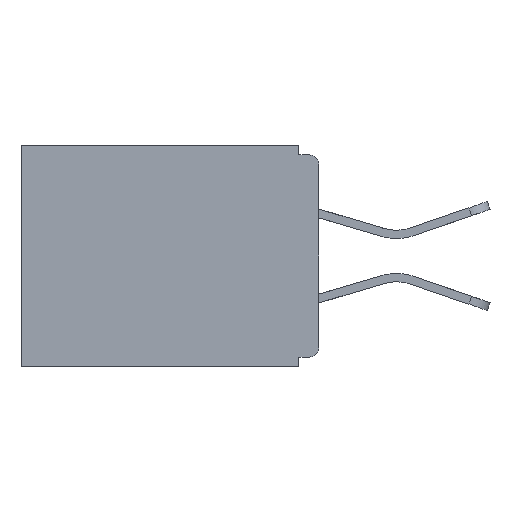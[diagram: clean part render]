
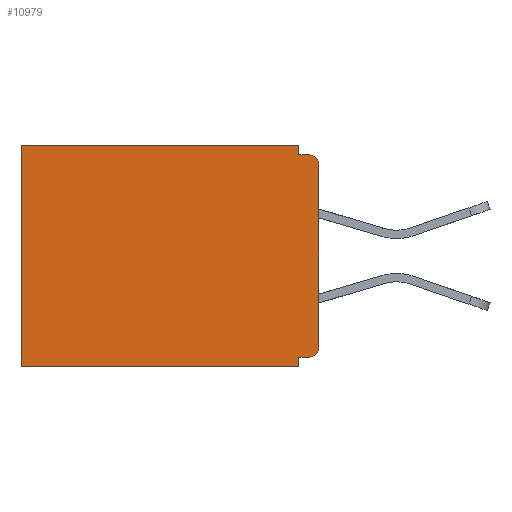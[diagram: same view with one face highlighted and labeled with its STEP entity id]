
A CAD part, left-side view. The second image highlights one B-rep face of the part: STEP entity #10979.
In plain terms, the highlighted planar face has unit normal (-1, 0, 0).
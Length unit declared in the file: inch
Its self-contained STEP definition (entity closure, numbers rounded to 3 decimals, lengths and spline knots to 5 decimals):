
#209 = CARTESIAN_POINT ( 'NONE',  ( 0.298, 0., 0. ) ) ;
#227 = ORIENTED_EDGE ( 'NONE', *, *, #17039, .T. ) ;
#592 = LINE ( 'NONE', #7194, #16999 ) ;
#690 = EDGE_CURVE ( 'NONE', #20075, #6422, #6167, .T. ) ;
#1209 = CARTESIAN_POINT ( 'NONE',  ( 0.298, 0.46, -0.343 ) ) ;
#1606 = EDGE_CURVE ( 'NONE', #6919, #14593, #592, .T. ) ;
#1772 = ORIENTED_EDGE ( 'NONE', *, *, #690, .T. ) ;
#1932 = DIRECTION ( 'NONE',  ( 0., 0., -1. ) ) ;
#1971 = CARTESIAN_POINT ( 'NONE',  ( 0.298, 0., -0.328 ) ) ;
#2287 = DIRECTION ( 'NONE',  ( 0., 0., -1. ) ) ;
#2556 = LINE ( 'NONE', #24312, #23766 ) ;
#2982 = CARTESIAN_POINT ( 'NONE',  ( 0.298, 0., 0. ) ) ;
#3265 = ORIENTED_EDGE ( 'NONE', *, *, #5584, .F. ) ;
#4301 = CARTESIAN_POINT ( 'NONE',  ( 0.298, 0.015, -0.03 ) ) ;
#4576 = VECTOR ( 'NONE', #20540, 39.37008 ) ;
#4629 = DIRECTION ( 'NONE',  ( 0., 0., -1. ) ) ;
#4659 = EDGE_CURVE ( 'NONE', #20075, #15726, #24919, .T. ) ;
#4704 = CARTESIAN_POINT ( 'NONE',  ( 0.298, 0.031, 0. ) ) ;
#5392 = FACE_OUTER_BOUND ( 'NONE', #14101, .T. ) ;
#5584 = EDGE_CURVE ( 'NONE', #16088, #6422, #20590, .T. ) ;
#5958 = ORIENTED_EDGE ( 'NONE', *, *, #4659, .F. ) ;
#6167 = CIRCLE ( 'NONE', #26015, 0.015 ) ;
#6249 = CARTESIAN_POINT ( 'NONE',  ( 0.298, 0.46, 0. ) ) ;
#6354 = VECTOR ( 'NONE', #13911, 39.37008 ) ;
#6369 = ORIENTED_EDGE ( 'NONE', *, *, #21008, .T. ) ;
#6422 = VERTEX_POINT ( 'NONE', #22270 ) ;
#6476 = CARTESIAN_POINT ( 'NONE',  ( 0.298, 0., -0.015 ) ) ;
#6669 = CARTESIAN_POINT ( 'NONE',  ( 0.298, 0.015, -0.328 ) ) ;
#6919 = VERTEX_POINT ( 'NONE', #22104 ) ;
#7194 = CARTESIAN_POINT ( 'NONE',  ( 0.298, 0., -0.343 ) ) ;
#7736 = VERTEX_POINT ( 'NONE', #6249 ) ;
#7957 = LINE ( 'NONE', #23876, #6354 ) ;
#8005 = LINE ( 'NONE', #2982, #18879 ) ;
#9027 = VERTEX_POINT ( 'NONE', #17617 ) ;
#10189 = DIRECTION ( 'NONE',  ( 0., 0., -1. ) ) ;
#10411 = DIRECTION ( 'NONE',  ( 0., 1., 0. ) ) ;
#10531 = PLANE ( 'NONE',  #12973 ) ;
#10979 = ADVANCED_FACE ( 'NONE', ( #5392 ), #10531, .F. ) ;
#11213 = LINE ( 'NONE', #6476, #12820 ) ;
#11377 = VECTOR ( 'NONE', #10411, 39.37008 ) ;
#11609 = CARTESIAN_POINT ( 'NONE',  ( 0.298, 0.031, -0.015 ) ) ;
#12205 = ORIENTED_EDGE ( 'NONE', *, *, #13034, .T. ) ;
#12239 = CARTESIAN_POINT ( 'NONE',  ( 0.298, 0.015, -0.313 ) ) ;
#12820 = VECTOR ( 'NONE', #18508, 39.37008 ) ;
#12973 = AXIS2_PLACEMENT_3D ( 'NONE', #209, #14638, #16970 ) ;
#13034 = EDGE_CURVE ( 'NONE', #16088, #9027, #21733, .T. ) ;
#13911 = DIRECTION ( 'NONE',  ( 0., 0., -1. ) ) ;
#14101 = EDGE_LOOP ( 'NONE', ( #12205, #18159, #20805, #227, #6369, #18441, #16629, #5958, #1772, #3265 ) ) ;
#14593 = VERTEX_POINT ( 'NONE', #1209 ) ;
#14638 = DIRECTION ( 'NONE',  ( 1., 0., 0. ) ) ;
#14910 = EDGE_CURVE ( 'NONE', #15726, #6919, #21263, .T. ) ;
#15726 = VERTEX_POINT ( 'NONE', #17563 ) ;
#16088 = VERTEX_POINT ( 'NONE', #19944 ) ;
#16100 = EDGE_CURVE ( 'NONE', #24744, #9027, #11213, .T. ) ;
#16577 = CARTESIAN_POINT ( 'NONE',  ( 0.298, 0.031, -0.343 ) ) ;
#16629 = ORIENTED_EDGE ( 'NONE', *, *, #14910, .F. ) ;
#16892 = VERTEX_POINT ( 'NONE', #4704 ) ;
#16970 = DIRECTION ( 'NONE',  ( 0., 0., -1. ) ) ;
#16999 = VECTOR ( 'NONE', #25496, 39.37008 ) ;
#17039 = EDGE_CURVE ( 'NONE', #16892, #7736, #8005, .T. ) ;
#17346 = DIRECTION ( 'NONE',  ( 0., 1., 0. ) ) ;
#17563 = CARTESIAN_POINT ( 'NONE',  ( 0.298, 0.031, -0.328 ) ) ;
#17617 = CARTESIAN_POINT ( 'NONE',  ( 0.298, 0.015, -0.015 ) ) ;
#18159 = ORIENTED_EDGE ( 'NONE', *, *, #16100, .F. ) ;
#18441 = ORIENTED_EDGE ( 'NONE', *, *, #1606, .F. ) ;
#18508 = DIRECTION ( 'NONE',  ( 0., -1., 0. ) ) ;
#18729 = CARTESIAN_POINT ( 'NONE',  ( 0.298, 0., 0. ) ) ;
#18879 = VECTOR ( 'NONE', #17346, 39.37008 ) ;
#19264 = VECTOR ( 'NONE', #2287, 39.37008 ) ;
#19934 = AXIS2_PLACEMENT_3D ( 'NONE', #4301, #24936, #4629 ) ;
#19944 = CARTESIAN_POINT ( 'NONE',  ( 0.298, 0., -0.03 ) ) ;
#20075 = VERTEX_POINT ( 'NONE', #6669 ) ;
#20540 = DIRECTION ( 'NONE',  ( 0., 0., -1. ) ) ;
#20590 = LINE ( 'NONE', #18729, #19264 ) ;
#20805 = ORIENTED_EDGE ( 'NONE', *, *, #22495, .F. ) ;
#21008 = EDGE_CURVE ( 'NONE', #7736, #14593, #2556, .T. ) ;
#21263 = LINE ( 'NONE', #16577, #4576 ) ;
#21733 = CIRCLE ( 'NONE', #19934, 0.015 ) ;
#22104 = CARTESIAN_POINT ( 'NONE',  ( 0.298, 0.031, -0.343 ) ) ;
#22270 = CARTESIAN_POINT ( 'NONE',  ( 0.298, 0., -0.313 ) ) ;
#22495 = EDGE_CURVE ( 'NONE', #16892, #24744, #7957, .T. ) ;
#23766 = VECTOR ( 'NONE', #1932, 39.37008 ) ;
#23876 = CARTESIAN_POINT ( 'NONE',  ( 0.298, 0.031, -0.343 ) ) ;
#24312 = CARTESIAN_POINT ( 'NONE',  ( 0.298, 0.46, 0. ) ) ;
#24744 = VERTEX_POINT ( 'NONE', #11609 ) ;
#24919 = LINE ( 'NONE', #1971, #11377 ) ;
#24936 = DIRECTION ( 'NONE',  ( -1., 0., 0. ) ) ;
#25496 = DIRECTION ( 'NONE',  ( 0., 1., 0. ) ) ;
#26015 = AXIS2_PLACEMENT_3D ( 'NONE', #12239, #26518, #10189 ) ;
#26518 = DIRECTION ( 'NONE',  ( -1., 0., 0. ) ) ;
